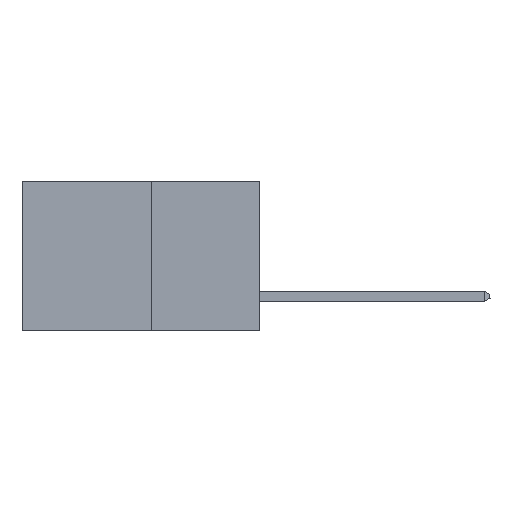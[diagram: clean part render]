
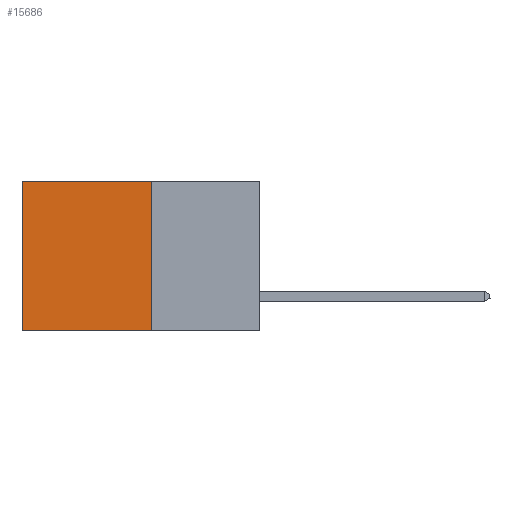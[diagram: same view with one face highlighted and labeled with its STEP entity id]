
A CAD part, left-side view. The second image highlights one B-rep face of the part: STEP entity #15686.
In plain terms, the highlighted planar face has unit normal (-1, 0, 0).
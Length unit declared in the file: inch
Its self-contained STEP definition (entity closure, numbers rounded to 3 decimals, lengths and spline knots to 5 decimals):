
#629 = EDGE_CURVE ( 'NONE', #2203, #6630, #7595, .T. ) ;
#745 = EDGE_CURVE ( 'NONE', #18970, #10659, #5238, .T. ) ;
#1602 = CARTESIAN_POINT ( 'NONE',  ( 0.277, 0.27, -0.37 ) ) ;
#1648 = AXIS2_PLACEMENT_3D ( 'NONE', #5338, #17226, #8372 ) ;
#2203 = VERTEX_POINT ( 'NONE', #9586 ) ;
#2263 = CARTESIAN_POINT ( 'NONE',  ( 0.277, 0.59, -0.37 ) ) ;
#2569 = FACE_OUTER_BOUND ( 'NONE', #8371, .T. ) ;
#2685 = EDGE_CURVE ( 'NONE', #2203, #18970, #9883, .T. ) ;
#2928 = DIRECTION ( 'NONE',  ( 0., 0., -1. ) ) ;
#3397 = CARTESIAN_POINT ( 'NONE',  ( 0.277, 0.27, -0.37 ) ) ;
#5238 = LINE ( 'NONE', #9315, #13307 ) ;
#5338 = CARTESIAN_POINT ( 'NONE',  ( 0.277, 0.27, -0.37 ) ) ;
#5727 = DIRECTION ( 'NONE',  ( 0., 0., -1. ) ) ;
#5981 = VECTOR ( 'NONE', #10489, 39.37008 ) ;
#6141 = EDGE_CURVE ( 'NONE', #6630, #10659, #6458, .T. ) ;
#6458 = LINE ( 'NONE', #10361, #5981 ) ;
#6630 = VERTEX_POINT ( 'NONE', #1602 ) ;
#7595 = LINE ( 'NONE', #3397, #14688 ) ;
#8371 = EDGE_LOOP ( 'NONE', ( #12545, #12581, #12656, #12688 ) ) ;
#8372 = DIRECTION ( 'NONE',  ( 0., 0., -1. ) ) ;
#9315 = CARTESIAN_POINT ( 'NONE',  ( 0.277, 0.59, -0.37 ) ) ;
#9586 = CARTESIAN_POINT ( 'NONE',  ( 0.277, 0.27, 0. ) ) ;
#9883 = LINE ( 'NONE', #13161, #10369 ) ;
#10361 = CARTESIAN_POINT ( 'NONE',  ( 0.277, 0.27, -0.37 ) ) ;
#10369 = VECTOR ( 'NONE', #13836, 39.37008 ) ;
#10489 = DIRECTION ( 'NONE',  ( 0., 1., 0. ) ) ;
#10579 = CARTESIAN_POINT ( 'NONE',  ( 0.277, 0.59, 0. ) ) ;
#10659 = VERTEX_POINT ( 'NONE', #2263 ) ;
#12545 = ORIENTED_EDGE ( 'NONE', *, *, #745, .T. ) ;
#12581 = ORIENTED_EDGE ( 'NONE', *, *, #6141, .F. ) ;
#12656 = ORIENTED_EDGE ( 'NONE', *, *, #629, .F. ) ;
#12688 = ORIENTED_EDGE ( 'NONE', *, *, #2685, .T. ) ;
#13161 = CARTESIAN_POINT ( 'NONE',  ( 0.277, 0.27, 0. ) ) ;
#13307 = VECTOR ( 'NONE', #2928, 39.37008 ) ;
#13836 = DIRECTION ( 'NONE',  ( 0., 1., 0. ) ) ;
#14688 = VECTOR ( 'NONE', #5727, 39.37008 ) ;
#15686 = ADVANCED_FACE ( 'NONE', ( #2569 ), #15810, .F. ) ;
#15810 = PLANE ( 'NONE',  #1648 ) ;
#17226 = DIRECTION ( 'NONE',  ( 1., 0., 0. ) ) ;
#18970 = VERTEX_POINT ( 'NONE', #10579 ) ;
